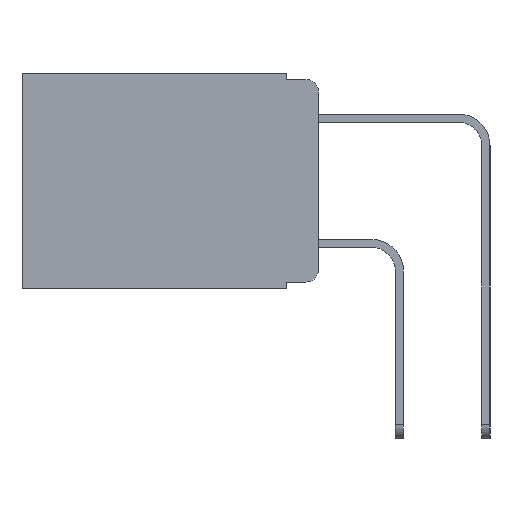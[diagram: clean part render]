
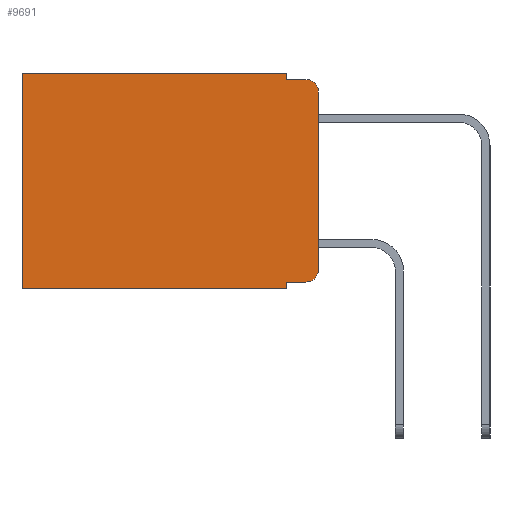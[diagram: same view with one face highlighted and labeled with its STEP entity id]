
A CAD part, left-side view. The second image highlights one B-rep face of the part: STEP entity #9691.
In plain terms, the highlighted planar face has unit normal (-1, 0, 0).
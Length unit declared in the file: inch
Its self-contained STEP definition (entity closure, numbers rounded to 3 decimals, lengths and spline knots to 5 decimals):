
#354 = VERTEX_POINT ( 'NONE', #3281 ) ;
#603 = FACE_OUTER_BOUND ( 'NONE', #1275, .T. ) ;
#755 = VERTEX_POINT ( 'NONE', #15258 ) ;
#798 = CARTESIAN_POINT ( 'NONE',  ( 0.298, 0.051, 0. ) ) ;
#818 = EDGE_CURVE ( 'NONE', #7678, #8347, #8310, .T. ) ;
#1046 = LINE ( 'NONE', #9701, #13832 ) ;
#1275 = EDGE_LOOP ( 'NONE', ( #12645, #1828, #5666, #9246, #14101, #13195, #2025, #14274, #12258, #5682 ) ) ;
#1443 = CIRCLE ( 'NONE', #10138, 0.02 ) ;
#1659 = CARTESIAN_POINT ( 'NONE',  ( 0.298, 0.051, -0.333 ) ) ;
#1739 = EDGE_CURVE ( 'NONE', #6890, #11899, #2387, .T. ) ;
#1828 = ORIENTED_EDGE ( 'NONE', *, *, #4368, .T. ) ;
#2025 = ORIENTED_EDGE ( 'NONE', *, *, #11375, .F. ) ;
#2298 = VECTOR ( 'NONE', #9867, 39.37008 ) ;
#2387 = LINE ( 'NONE', #9226, #5435 ) ;
#2492 = LINE ( 'NONE', #8268, #11928 ) ;
#2623 = EDGE_CURVE ( 'NONE', #5602, #5228, #7103, .T. ) ;
#2666 = CARTESIAN_POINT ( 'NONE',  ( 0.298, 0., 0. ) ) ;
#2699 = CARTESIAN_POINT ( 'NONE',  ( 0.298, 0.051, 0. ) ) ;
#3281 = CARTESIAN_POINT ( 'NONE',  ( 0.298, 0., -0.03 ) ) ;
#3377 = CARTESIAN_POINT ( 'NONE',  ( 0.298, 0.051, 0. ) ) ;
#3487 = EDGE_CURVE ( 'NONE', #5228, #755, #1046, .T. ) ;
#3970 = DIRECTION ( 'NONE',  ( 0., 0., -1. ) ) ;
#4368 = EDGE_CURVE ( 'NONE', #354, #755, #1443, .T. ) ;
#4938 = CARTESIAN_POINT ( 'NONE',  ( 0.298, 0.02, -0.333 ) ) ;
#5074 = VECTOR ( 'NONE', #10884, 39.37008 ) ;
#5228 = VERTEX_POINT ( 'NONE', #7275 ) ;
#5435 = VECTOR ( 'NONE', #6475, 39.37008 ) ;
#5602 = VERTEX_POINT ( 'NONE', #3377 ) ;
#5666 = ORIENTED_EDGE ( 'NONE', *, *, #3487, .F. ) ;
#5682 = ORIENTED_EDGE ( 'NONE', *, *, #15124, .T. ) ;
#5921 = CARTESIAN_POINT ( 'NONE',  ( 0.298, 0.473, -0.343 ) ) ;
#6196 = DIRECTION ( 'NONE',  ( -1., 0., 0. ) ) ;
#6401 = VECTOR ( 'NONE', #3970, 39.37008 ) ;
#6475 = DIRECTION ( 'NONE',  ( 0., 0., -1. ) ) ;
#6764 = DIRECTION ( 'NONE',  ( -1., 0., 0. ) ) ;
#6882 = EDGE_CURVE ( 'NONE', #354, #13182, #9571, .T. ) ;
#6890 = VERTEX_POINT ( 'NONE', #12496 ) ;
#6996 = CARTESIAN_POINT ( 'NONE',  ( 0.298, 0.02, -0.03 ) ) ;
#7101 = AXIS2_PLACEMENT_3D ( 'NONE', #11671, #15196, #8142 ) ;
#7103 = LINE ( 'NONE', #798, #9531 ) ;
#7275 = CARTESIAN_POINT ( 'NONE',  ( 0.298, 0.051, -0.01 ) ) ;
#7342 = DIRECTION ( 'NONE',  ( 0., 0., -1. ) ) ;
#7678 = VERTEX_POINT ( 'NONE', #1659 ) ;
#8042 = CIRCLE ( 'NONE', #11005, 0.02 ) ;
#8142 = DIRECTION ( 'NONE',  ( 0., 0., -1. ) ) ;
#8268 = CARTESIAN_POINT ( 'NONE',  ( 0.298, 0.051, -0.333 ) ) ;
#8310 = LINE ( 'NONE', #2699, #5074 ) ;
#8347 = VERTEX_POINT ( 'NONE', #12871 ) ;
#8739 = DIRECTION ( 'NONE',  ( 0., -1., 0. ) ) ;
#9166 = DIRECTION ( 'NONE',  ( 0., 1., 0. ) ) ;
#9226 = CARTESIAN_POINT ( 'NONE',  ( 0.298, 0.473, 0. ) ) ;
#9246 = ORIENTED_EDGE ( 'NONE', *, *, #2623, .F. ) ;
#9531 = VECTOR ( 'NONE', #12599, 39.37008 ) ;
#9571 = LINE ( 'NONE', #2666, #6401 ) ;
#9616 = LINE ( 'NONE', #11564, #12834 ) ;
#9691 = ADVANCED_FACE ( 'NONE', ( #603 ), #14064, .F. ) ;
#9701 = CARTESIAN_POINT ( 'NONE',  ( 0.298, 0.051, -0.01 ) ) ;
#9867 = DIRECTION ( 'NONE',  ( 0., 1., 0. ) ) ;
#9980 = EDGE_CURVE ( 'NONE', #5602, #6890, #12120, .T. ) ;
#10138 = AXIS2_PLACEMENT_3D ( 'NONE', #6996, #6196, #7342 ) ;
#10643 = DIRECTION ( 'NONE',  ( 0., -1., 0. ) ) ;
#10884 = DIRECTION ( 'NONE',  ( 0., 0., -1. ) ) ;
#11005 = AXIS2_PLACEMENT_3D ( 'NONE', #13931, #6764, #15063 ) ;
#11375 = EDGE_CURVE ( 'NONE', #8347, #11899, #9616, .T. ) ;
#11564 = CARTESIAN_POINT ( 'NONE',  ( 0.298, 0., -0.343 ) ) ;
#11671 = CARTESIAN_POINT ( 'NONE',  ( 0.298, 0., 0. ) ) ;
#11899 = VERTEX_POINT ( 'NONE', #5921 ) ;
#11928 = VECTOR ( 'NONE', #10643, 39.37008 ) ;
#11997 = CARTESIAN_POINT ( 'NONE',  ( 0.298, 0., -0.313 ) ) ;
#12120 = LINE ( 'NONE', #14611, #2298 ) ;
#12258 = ORIENTED_EDGE ( 'NONE', *, *, #15860, .T. ) ;
#12496 = CARTESIAN_POINT ( 'NONE',  ( 0.298, 0.473, 0. ) ) ;
#12599 = DIRECTION ( 'NONE',  ( 0., 0., -1. ) ) ;
#12645 = ORIENTED_EDGE ( 'NONE', *, *, #6882, .F. ) ;
#12834 = VECTOR ( 'NONE', #9166, 39.37008 ) ;
#12871 = CARTESIAN_POINT ( 'NONE',  ( 0.298, 0.051, -0.343 ) ) ;
#13182 = VERTEX_POINT ( 'NONE', #11997 ) ;
#13195 = ORIENTED_EDGE ( 'NONE', *, *, #1739, .T. ) ;
#13832 = VECTOR ( 'NONE', #8739, 39.37008 ) ;
#13931 = CARTESIAN_POINT ( 'NONE',  ( 0.298, 0.02, -0.313 ) ) ;
#14064 = PLANE ( 'NONE',  #7101 ) ;
#14101 = ORIENTED_EDGE ( 'NONE', *, *, #9980, .T. ) ;
#14274 = ORIENTED_EDGE ( 'NONE', *, *, #818, .F. ) ;
#14371 = VERTEX_POINT ( 'NONE', #4938 ) ;
#14611 = CARTESIAN_POINT ( 'NONE',  ( 0.298, 0., 0. ) ) ;
#15063 = DIRECTION ( 'NONE',  ( 0., 0., -1. ) ) ;
#15124 = EDGE_CURVE ( 'NONE', #14371, #13182, #8042, .T. ) ;
#15196 = DIRECTION ( 'NONE',  ( 1., 0., 0. ) ) ;
#15258 = CARTESIAN_POINT ( 'NONE',  ( 0.298, 0.02, -0.01 ) ) ;
#15860 = EDGE_CURVE ( 'NONE', #7678, #14371, #2492, .T. ) ;
